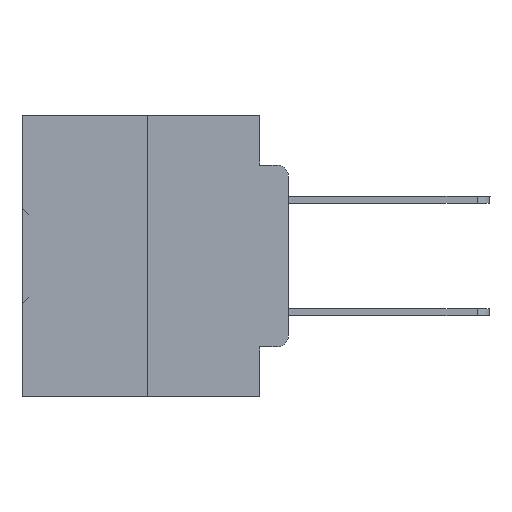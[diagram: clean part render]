
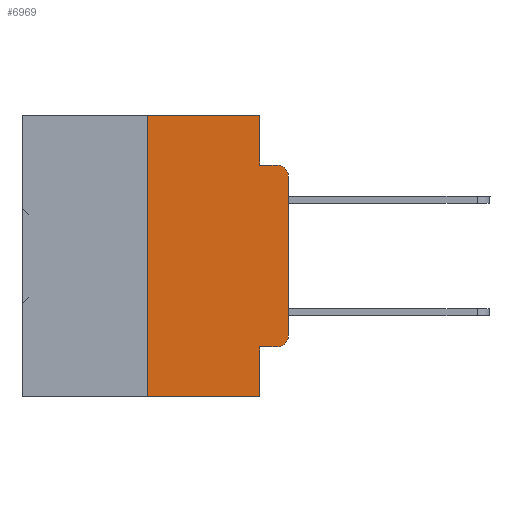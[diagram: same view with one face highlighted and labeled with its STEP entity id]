
A CAD part, left-side view. The second image highlights one B-rep face of the part: STEP entity #6969.
In plain terms, the highlighted planar face has unit normal (-1, 0, 0).
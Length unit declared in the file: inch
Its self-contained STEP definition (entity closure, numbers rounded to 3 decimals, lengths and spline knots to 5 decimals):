
#126 = CARTESIAN_POINT ( 'NONE',  ( 0., 0.051, -0.0885 ) ) ;
#338 = ORIENTED_EDGE ( 'NONE', *, *, #31457, .F. ) ;
#683 = CARTESIAN_POINT ( 'NONE',  ( 0., 0.02, -0.3915 ) ) ;
#993 = CIRCLE ( 'NONE', #17515, 0.02 ) ;
#1047 = CARTESIAN_POINT ( 'NONE',  ( 0., 0.02, -0.0885 ) ) ;
#1072 = DIRECTION ( 'NONE',  ( 1., 0., 0. ) ) ;
#1124 = ORIENTED_EDGE ( 'NONE', *, *, #28401, .F. ) ;
#1490 = VECTOR ( 'NONE', #20829, 39.37008 ) ;
#1959 = EDGE_LOOP ( 'NONE', ( #15584, #30327, #38991, #1124, #33407, #17054, #20336, #338, #29641, #36920 ) ) ;
#2722 = DIRECTION ( 'NONE',  ( 0., -1., 0. ) ) ;
#3424 = CARTESIAN_POINT ( 'NONE',  ( 0., 0.25, -0.5 ) ) ;
#5482 = VERTEX_POINT ( 'NONE', #3424 ) ;
#5704 = CARTESIAN_POINT ( 'NONE',  ( 0., 0.051, -0.4115 ) ) ;
#5931 = LINE ( 'NONE', #11899, #1490 ) ;
#6079 = DIRECTION ( 'NONE',  ( 0., -1., 0. ) ) ;
#6969 = ADVANCED_FACE ( 'NONE', ( #22524 ), #7230, .F. ) ;
#7230 = PLANE ( 'NONE',  #35408 ) ;
#8249 = DIRECTION ( 'NONE',  ( 0., 0., 1. ) ) ;
#8388 = DIRECTION ( 'NONE',  ( 0., -1., 0. ) ) ;
#8444 = LINE ( 'NONE', #26147, #27238 ) ;
#8689 = DIRECTION ( 'NONE',  ( 0., 0., -1. ) ) ;
#8873 = LINE ( 'NONE', #126, #34029 ) ;
#8927 = VERTEX_POINT ( 'NONE', #33348 ) ;
#9543 = VERTEX_POINT ( 'NONE', #34293 ) ;
#9696 = EDGE_CURVE ( 'NONE', #12757, #8927, #8444, .T. ) ;
#9734 = CARTESIAN_POINT ( 'NONE',  ( 0., 0.051, 0. ) ) ;
#11899 = CARTESIAN_POINT ( 'NONE',  ( 0., 0.25, 0. ) ) ;
#12757 = VERTEX_POINT ( 'NONE', #19893 ) ;
#12824 = EDGE_CURVE ( 'NONE', #19198, #13274, #32607, .T. ) ;
#12950 = CARTESIAN_POINT ( 'NONE',  ( 0., 0.02, -0.4115 ) ) ;
#12968 = VECTOR ( 'NONE', #6079, 39.37008 ) ;
#13274 = VERTEX_POINT ( 'NONE', #35926 ) ;
#15584 = ORIENTED_EDGE ( 'NONE', *, *, #9696, .T. ) ;
#16394 = AXIS2_PLACEMENT_3D ( 'NONE', #24909, #18920, #37431 ) ;
#16794 = EDGE_CURVE ( 'NONE', #5482, #9543, #18598, .T. ) ;
#17054 = ORIENTED_EDGE ( 'NONE', *, *, #23228, .F. ) ;
#17515 = AXIS2_PLACEMENT_3D ( 'NONE', #683, #33661, #18372 ) ;
#18372 = DIRECTION ( 'NONE',  ( 0., 0., -1. ) ) ;
#18598 = LINE ( 'NONE', #21960, #31188 ) ;
#18920 = DIRECTION ( 'NONE',  ( -1., 0., 0. ) ) ;
#19198 = VERTEX_POINT ( 'NONE', #34803 ) ;
#19536 = DIRECTION ( 'NONE',  ( 0., 0., -1. ) ) ;
#19893 = CARTESIAN_POINT ( 'NONE',  ( 0., 0., -0.3915 ) ) ;
#20336 = ORIENTED_EDGE ( 'NONE', *, *, #16794, .T. ) ;
#20829 = DIRECTION ( 'NONE',  ( 0., 0., 1. ) ) ;
#21960 = CARTESIAN_POINT ( 'NONE',  ( 0., 0.473, -0.5 ) ) ;
#22524 = FACE_OUTER_BOUND ( 'NONE', #1959, .T. ) ;
#22874 = VECTOR ( 'NONE', #8689, 39.37008 ) ;
#23228 = EDGE_CURVE ( 'NONE', #5482, #19198, #5931, .T. ) ;
#23454 = VECTOR ( 'NONE', #34577, 39.37008 ) ;
#23687 = VERTEX_POINT ( 'NONE', #12950 ) ;
#23798 = LINE ( 'NONE', #24201, #22874 ) ;
#24201 = CARTESIAN_POINT ( 'NONE',  ( 0., 0.051, 0. ) ) ;
#24909 = CARTESIAN_POINT ( 'NONE',  ( 0., 0.02, -0.1085 ) ) ;
#25064 = VECTOR ( 'NONE', #8388, 39.37008 ) ;
#26080 = EDGE_CURVE ( 'NONE', #30128, #23687, #33288, .T. ) ;
#26147 = CARTESIAN_POINT ( 'NONE',  ( 0., 0., 0. ) ) ;
#26964 = CARTESIAN_POINT ( 'NONE',  ( 0., 0.051, -0.4115 ) ) ;
#27238 = VECTOR ( 'NONE', #8249, 39.37008 ) ;
#27444 = CARTESIAN_POINT ( 'NONE',  ( 0., 0.473, 0. ) ) ;
#28060 = EDGE_CURVE ( 'NONE', #8927, #32163, #29111, .T. ) ;
#28294 = CARTESIAN_POINT ( 'NONE',  ( 0., 0.473, 0. ) ) ;
#28401 = EDGE_CURVE ( 'NONE', #13274, #33190, #31373, .T. ) ;
#29111 = CIRCLE ( 'NONE', #16394, 0.02 ) ;
#29641 = ORIENTED_EDGE ( 'NONE', *, *, #26080, .T. ) ;
#29968 = CARTESIAN_POINT ( 'NONE',  ( 0., 0.051, -0.0885 ) ) ;
#30128 = VERTEX_POINT ( 'NONE', #5704 ) ;
#30327 = ORIENTED_EDGE ( 'NONE', *, *, #28060, .T. ) ;
#31188 = VECTOR ( 'NONE', #34496, 39.37008 ) ;
#31373 = LINE ( 'NONE', #9734, #23454 ) ;
#31457 = EDGE_CURVE ( 'NONE', #30128, #9543, #23798, .T. ) ;
#32163 = VERTEX_POINT ( 'NONE', #1047 ) ;
#32607 = LINE ( 'NONE', #27444, #25064 ) ;
#33190 = VERTEX_POINT ( 'NONE', #29968 ) ;
#33288 = LINE ( 'NONE', #26964, #12968 ) ;
#33348 = CARTESIAN_POINT ( 'NONE',  ( 0., 0., -0.1085 ) ) ;
#33407 = ORIENTED_EDGE ( 'NONE', *, *, #12824, .F. ) ;
#33661 = DIRECTION ( 'NONE',  ( -1., 0., 0. ) ) ;
#33759 = EDGE_CURVE ( 'NONE', #23687, #12757, #993, .T. ) ;
#34029 = VECTOR ( 'NONE', #2722, 39.37008 ) ;
#34293 = CARTESIAN_POINT ( 'NONE',  ( 0., 0.051, -0.5 ) ) ;
#34496 = DIRECTION ( 'NONE',  ( 0., -1., 0. ) ) ;
#34577 = DIRECTION ( 'NONE',  ( 0., 0., -1. ) ) ;
#34803 = CARTESIAN_POINT ( 'NONE',  ( 0., 0.25, 0. ) ) ;
#35408 = AXIS2_PLACEMENT_3D ( 'NONE', #28294, #1072, #19536 ) ;
#35926 = CARTESIAN_POINT ( 'NONE',  ( 0., 0.051, 0. ) ) ;
#36201 = EDGE_CURVE ( 'NONE', #33190, #32163, #8873, .T. ) ;
#36920 = ORIENTED_EDGE ( 'NONE', *, *, #33759, .T. ) ;
#37431 = DIRECTION ( 'NONE',  ( 0., 0., -1. ) ) ;
#38991 = ORIENTED_EDGE ( 'NONE', *, *, #36201, .F. ) ;
